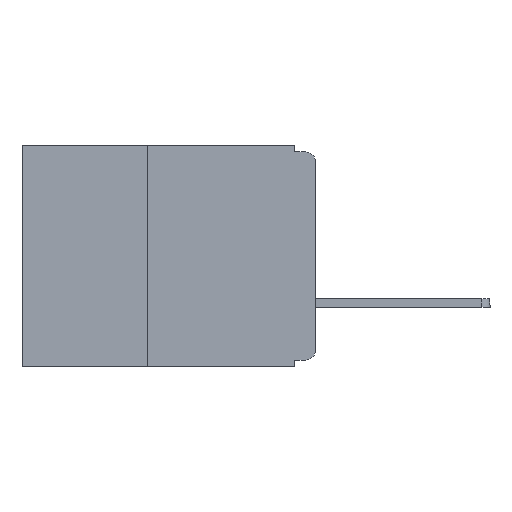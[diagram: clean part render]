
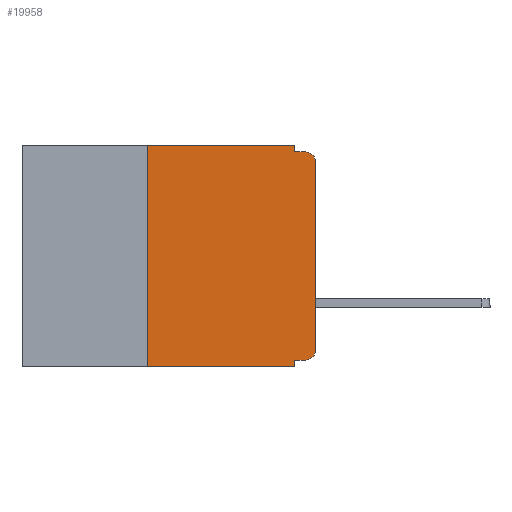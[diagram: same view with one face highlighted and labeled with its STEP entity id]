
A CAD part, left-side view. The second image highlights one B-rep face of the part: STEP entity #19958.
In plain terms, the highlighted planar face has unit normal (-1, 0, 0).
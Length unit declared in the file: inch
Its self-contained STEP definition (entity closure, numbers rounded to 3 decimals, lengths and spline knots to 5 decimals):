
#527 = VERTEX_POINT ( 'NONE', #12643 ) ;
#777 = EDGE_CURVE ( 'NONE', #9599, #2417, #16272, .T. ) ;
#1019 = VERTEX_POINT ( 'NONE', #17715 ) ;
#1340 = VECTOR ( 'NONE', #23247, 39.37008 ) ;
#2108 = AXIS2_PLACEMENT_3D ( 'NONE', #2864, #16103, #4786 ) ;
#2235 = ORIENTED_EDGE ( 'NONE', *, *, #21620, .F. ) ;
#2417 = VERTEX_POINT ( 'NONE', #18076 ) ;
#2451 = CARTESIAN_POINT ( 'NONE',  ( 0., 0.437, 0. ) ) ;
#2570 = VECTOR ( 'NONE', #11788, 39.37008 ) ;
#2864 = CARTESIAN_POINT ( 'NONE',  ( 0., 0.015, -0.025 ) ) ;
#3611 = CARTESIAN_POINT ( 'NONE',  ( 0., 0., 0. ) ) ;
#3784 = LINE ( 'NONE', #9858, #2570 ) ;
#4350 = VERTEX_POINT ( 'NONE', #20212 ) ;
#4786 = DIRECTION ( 'NONE',  ( 0., 0., -1. ) ) ;
#5503 = DIRECTION ( 'NONE',  ( 0., 0., 1. ) ) ;
#5524 = DIRECTION ( 'NONE',  ( 0., 0., -1. ) ) ;
#5526 = ORIENTED_EDGE ( 'NONE', *, *, #777, .F. ) ;
#5823 = VECTOR ( 'NONE', #5503, 39.37008 ) ;
#6045 = AXIS2_PLACEMENT_3D ( 'NONE', #7622, #20866, #9493 ) ;
#6187 = VECTOR ( 'NONE', #23149, 39.37008 ) ;
#6660 = LINE ( 'NONE', #18020, #11087 ) ;
#6947 = ORIENTED_EDGE ( 'NONE', *, *, #9628, .T. ) ;
#7110 = EDGE_CURVE ( 'NONE', #527, #2417, #22517, .T. ) ;
#7232 = LINE ( 'NONE', #24324, #11681 ) ;
#7483 = DIRECTION ( 'NONE',  ( -1., 0., 0. ) ) ;
#7622 = CARTESIAN_POINT ( 'NONE',  ( 0., 0.437, 0. ) ) ;
#7900 = ORIENTED_EDGE ( 'NONE', *, *, #15145, .T. ) ;
#8445 = VERTEX_POINT ( 'NONE', #20413 ) ;
#8560 = DIRECTION ( 'NONE',  ( 0., 0., 1. ) ) ;
#9169 = CARTESIAN_POINT ( 'NONE',  ( 0., 0.031, -0.01 ) ) ;
#9250 = CARTESIAN_POINT ( 'NONE',  ( 0., 0.031, 0. ) ) ;
#9285 = ORIENTED_EDGE ( 'NONE', *, *, #7110, .T. ) ;
#9493 = DIRECTION ( 'NONE',  ( 0., 0., -1. ) ) ;
#9599 = VERTEX_POINT ( 'NONE', #9169 ) ;
#9628 = EDGE_CURVE ( 'NONE', #19704, #527, #10820, .T. ) ;
#9635 = VERTEX_POINT ( 'NONE', #9250 ) ;
#9858 = CARTESIAN_POINT ( 'NONE',  ( 0., 0., -0.32 ) ) ;
#10781 = EDGE_CURVE ( 'NONE', #1019, #19704, #19104, .T. ) ;
#10820 = LINE ( 'NONE', #3611, #5823 ) ;
#10914 = FACE_OUTER_BOUND ( 'NONE', #16731, .T. ) ;
#11087 = VECTOR ( 'NONE', #8560, 39.37008 ) ;
#11346 = VERTEX_POINT ( 'NONE', #14793 ) ;
#11424 = LINE ( 'NONE', #2451, #1340 ) ;
#11668 = AXIS2_PLACEMENT_3D ( 'NONE', #18826, #7483, #20738 ) ;
#11681 = VECTOR ( 'NONE', #5524, 39.37008 ) ;
#11788 = DIRECTION ( 'NONE',  ( 0., 1., 0. ) ) ;
#12458 = CARTESIAN_POINT ( 'NONE',  ( 0., 0., -0.305 ) ) ;
#12643 = CARTESIAN_POINT ( 'NONE',  ( 0., 0., -0.025 ) ) ;
#12708 = EDGE_CURVE ( 'NONE', #9635, #9599, #16843, .T. ) ;
#13092 = CARTESIAN_POINT ( 'NONE',  ( 0., 0.031, -0.32 ) ) ;
#14668 = ORIENTED_EDGE ( 'NONE', *, *, #21691, .F. ) ;
#14793 = CARTESIAN_POINT ( 'NONE',  ( 0., 0.25, -0.33 ) ) ;
#14860 = EDGE_CURVE ( 'NONE', #20459, #8445, #7232, .T. ) ;
#15145 = EDGE_CURVE ( 'NONE', #11346, #8445, #21996, .T. ) ;
#16103 = DIRECTION ( 'NONE',  ( -1., 0., 0. ) ) ;
#16253 = ORIENTED_EDGE ( 'NONE', *, *, #10781, .T. ) ;
#16272 = LINE ( 'NONE', #23317, #6187 ) ;
#16731 = EDGE_LOOP ( 'NONE', ( #6947, #9285, #5526, #23141, #14668, #23376, #7900, #22679, #2235, #16253 ) ) ;
#16843 = LINE ( 'NONE', #17689, #21255 ) ;
#17689 = CARTESIAN_POINT ( 'NONE',  ( 0., 0.031, 0. ) ) ;
#17715 = CARTESIAN_POINT ( 'NONE',  ( 0., 0.015, -0.32 ) ) ;
#18020 = CARTESIAN_POINT ( 'NONE',  ( 0., 0.25, -0.33 ) ) ;
#18076 = CARTESIAN_POINT ( 'NONE',  ( 0., 0.015, -0.01 ) ) ;
#18826 = CARTESIAN_POINT ( 'NONE',  ( 0., 0.015, -0.305 ) ) ;
#19104 = CIRCLE ( 'NONE', #11668, 0.015 ) ;
#19597 = DIRECTION ( 'NONE',  ( 0., 0., -1. ) ) ;
#19704 = VERTEX_POINT ( 'NONE', #12458 ) ;
#19823 = CARTESIAN_POINT ( 'NONE',  ( 0., 0.437, -0.33 ) ) ;
#19958 = ADVANCED_FACE ( 'NONE', ( #10914 ), #20785, .F. ) ;
#20212 = CARTESIAN_POINT ( 'NONE',  ( 0., 0.25, 0. ) ) ;
#20413 = CARTESIAN_POINT ( 'NONE',  ( 0., 0.031, -0.33 ) ) ;
#20459 = VERTEX_POINT ( 'NONE', #13092 ) ;
#20738 = DIRECTION ( 'NONE',  ( 0., 0., -1. ) ) ;
#20785 = PLANE ( 'NONE',  #6045 ) ;
#20851 = VECTOR ( 'NONE', #21689, 39.37008 ) ;
#20866 = DIRECTION ( 'NONE',  ( 1., 0., 0. ) ) ;
#21255 = VECTOR ( 'NONE', #19597, 39.37008 ) ;
#21620 = EDGE_CURVE ( 'NONE', #1019, #20459, #3784, .T. ) ;
#21689 = DIRECTION ( 'NONE',  ( 0., -1., 0. ) ) ;
#21691 = EDGE_CURVE ( 'NONE', #4350, #9635, #11424, .T. ) ;
#21996 = LINE ( 'NONE', #19823, #20851 ) ;
#22517 = CIRCLE ( 'NONE', #2108, 0.015 ) ;
#22679 = ORIENTED_EDGE ( 'NONE', *, *, #14860, .F. ) ;
#22978 = EDGE_CURVE ( 'NONE', #11346, #4350, #6660, .T. ) ;
#23141 = ORIENTED_EDGE ( 'NONE', *, *, #12708, .F. ) ;
#23149 = DIRECTION ( 'NONE',  ( 0., -1., 0. ) ) ;
#23247 = DIRECTION ( 'NONE',  ( 0., -1., 0. ) ) ;
#23317 = CARTESIAN_POINT ( 'NONE',  ( 0., 0., -0.01 ) ) ;
#23376 = ORIENTED_EDGE ( 'NONE', *, *, #22978, .F. ) ;
#24324 = CARTESIAN_POINT ( 'NONE',  ( 0., 0.031, -0.33 ) ) ;
